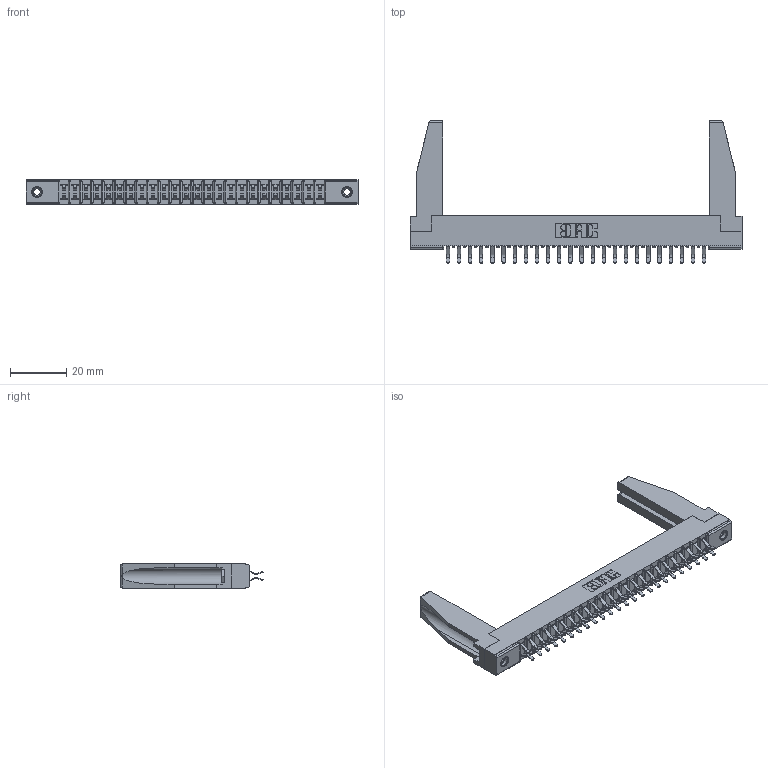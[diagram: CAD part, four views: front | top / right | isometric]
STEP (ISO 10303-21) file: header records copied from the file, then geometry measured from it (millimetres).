
FILE_DESCRIPTION (( 'STEP AP203' ), '1' );
FILE_NAME ('307-048-556-278.STEP', '2019-09-06T10:14:06', ( '' ), ( '' ), 'SwSTEP 2.0', 'SolidWorks 2016', '' );
FILE_SCHEMA (( 'CONFIG_CONTROL_DESIGN' ));
Length unit declared in the file: inch
Products named in the file (5): 307-048-556-278; 345-250-001_345-250-001-102; 307 Part_.156 Dia Mounting Holes; 307-220-078; 307-290-001_556
Assembly tree (53 placements, depth 2):
  307-048-556-278
    307 Part_.156 Dia Mounting Holes
    307-290-001_556  x48
    307-220-078  x2
    345-250-001_345-250-001-102  x2
Bounding box: 118.11 x 50.67 x 8.71 mm (x, y, z)
Volume: 11710.1 mm3; surface area: 17510 mm2
Topology: 53 solids, 53 shells, 2673 faces, 7469 edges, 4838 vertices
Faces by surface type: plane 1738, cylinder 869, sphere 50, cone 12, torus 4
Entity records: 26105 total; most frequent: CARTESIAN_POINT 4286, ORIENTED_EDGE 4204, DIRECTION 4160, EDGE_CURVE 2102, LINE 1608, VECTOR 1608, VERTEX_POINT 1360, AXIS2_PLACEMENT_3D 1276
